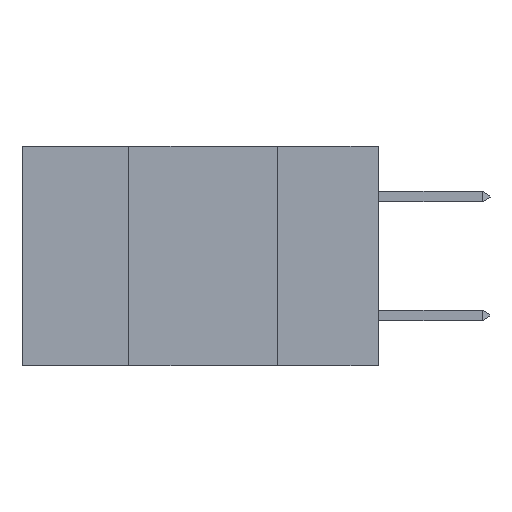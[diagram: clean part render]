
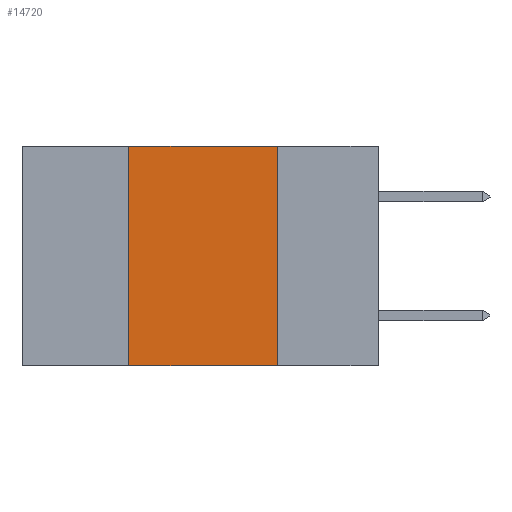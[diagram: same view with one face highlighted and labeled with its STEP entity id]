
A CAD part, left-side view. The second image highlights one B-rep face of the part: STEP entity #14720.
In plain terms, the highlighted planar face has unit normal (-1, 0, 0).
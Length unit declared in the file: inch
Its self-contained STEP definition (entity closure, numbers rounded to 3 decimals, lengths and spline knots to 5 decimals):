
#416 = LINE ( 'NONE', #4803, #9376 ) ;
#1473 = CARTESIAN_POINT ( 'NONE',  ( 0., 0.42, 0. ) ) ;
#1700 = CARTESIAN_POINT ( 'NONE',  ( 0., 0.17, 0. ) ) ;
#4394 = FACE_OUTER_BOUND ( 'NONE', #4910, .T. ) ;
#4618 = PLANE ( 'NONE',  #5082 ) ;
#4702 = DIRECTION ( 'NONE',  ( 0., 0., 1. ) ) ;
#4803 = CARTESIAN_POINT ( 'NONE',  ( 0., 0.6, 0. ) ) ;
#4910 = EDGE_LOOP ( 'NONE', ( #12503, #15028, #6212, #20722 ) ) ;
#5082 = AXIS2_PLACEMENT_3D ( 'NONE', #9695, #20894, #11369 ) ;
#5456 = VECTOR ( 'NONE', #4702, 39.37008 ) ;
#5964 = DIRECTION ( 'NONE',  ( 0., -1., 0. ) ) ;
#6186 = VERTEX_POINT ( 'NONE', #1473 ) ;
#6212 = ORIENTED_EDGE ( 'NONE', *, *, #14139, .F. ) ;
#6524 = DIRECTION ( 'NONE',  ( 0., -1., 0. ) ) ;
#6548 = LINE ( 'NONE', #13034, #5456 ) ;
#6774 = DIRECTION ( 'NONE',  ( 0., 0., -1. ) ) ;
#7365 = VECTOR ( 'NONE', #6774, 39.37008 ) ;
#8659 = CARTESIAN_POINT ( 'NONE',  ( 0., 0.42, -0.37 ) ) ;
#9138 = VECTOR ( 'NONE', #5964, 39.37008 ) ;
#9376 = VECTOR ( 'NONE', #6524, 39.37008 ) ;
#9695 = CARTESIAN_POINT ( 'NONE',  ( 0., 0.6, 0. ) ) ;
#10852 = EDGE_CURVE ( 'NONE', #12222, #20426, #16595, .T. ) ;
#11369 = DIRECTION ( 'NONE',  ( 0., 0., -1. ) ) ;
#11968 = EDGE_CURVE ( 'NONE', #12395, #20426, #13523, .T. ) ;
#12222 = VERTEX_POINT ( 'NONE', #21112 ) ;
#12395 = VERTEX_POINT ( 'NONE', #8659 ) ;
#12503 = ORIENTED_EDGE ( 'NONE', *, *, #10852, .F. ) ;
#13034 = CARTESIAN_POINT ( 'NONE',  ( 0., 0.42, 0. ) ) ;
#13523 = LINE ( 'NONE', #14254, #9138 ) ;
#14139 = EDGE_CURVE ( 'NONE', #12395, #6186, #6548, .T. ) ;
#14254 = CARTESIAN_POINT ( 'NONE',  ( 0., 0.6, -0.37 ) ) ;
#14720 = ADVANCED_FACE ( 'NONE', ( #4394 ), #4618, .F. ) ;
#15028 = ORIENTED_EDGE ( 'NONE', *, *, #15215, .F. ) ;
#15215 = EDGE_CURVE ( 'NONE', #6186, #12222, #416, .T. ) ;
#16595 = LINE ( 'NONE', #1700, #7365 ) ;
#20168 = CARTESIAN_POINT ( 'NONE',  ( 0., 0.17, -0.37 ) ) ;
#20426 = VERTEX_POINT ( 'NONE', #20168 ) ;
#20722 = ORIENTED_EDGE ( 'NONE', *, *, #11968, .T. ) ;
#20894 = DIRECTION ( 'NONE',  ( 1., 0., 0. ) ) ;
#21112 = CARTESIAN_POINT ( 'NONE',  ( 0., 0.17, 0. ) ) ;
